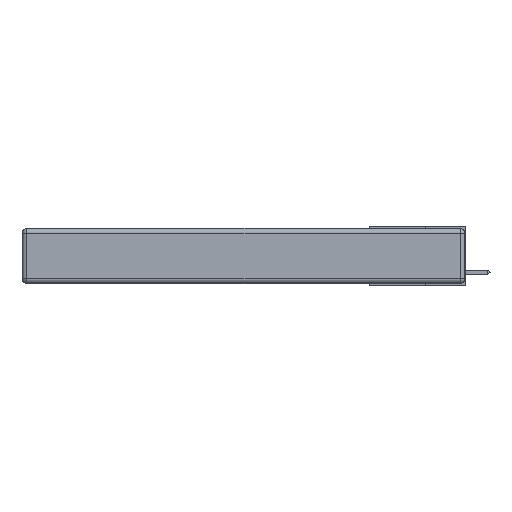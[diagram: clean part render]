
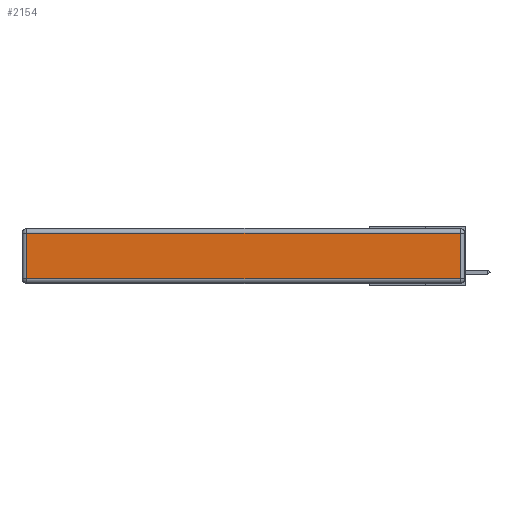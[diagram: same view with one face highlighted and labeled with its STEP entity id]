
A CAD part, left-side view. The second image highlights one B-rep face of the part: STEP entity #2154.
In plain terms, the highlighted planar face has unit normal (-1, 0, 0).
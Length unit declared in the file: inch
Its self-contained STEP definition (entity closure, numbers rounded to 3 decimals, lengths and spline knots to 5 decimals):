
#38 = CARTESIAN_POINT ( 'NONE',  ( 0., 2.75, -0.03 ) ) ;
#45 = CARTESIAN_POINT ( 'NONE',  ( 0., 0.03, -0.03 ) ) ;
#104 = DIRECTION ( 'NONE',  ( 0., 0., 1. ) ) ;
#1548 = VERTEX_POINT ( 'NONE', #6568 ) ;
#2064 = EDGE_LOOP ( 'NONE', ( #19879, #19993, #3849, #15967 ) ) ;
#2154 = ADVANCED_FACE ( 'NONE', ( #9152 ), #9570, .T. ) ;
#2314 = EDGE_CURVE ( 'NONE', #6201, #13058, #3477, .T. ) ;
#3466 = AXIS2_PLACEMENT_3D ( 'NONE', #19327, #9842, #104 ) ;
#3477 = LINE ( 'NONE', #8336, #7214 ) ;
#3849 = ORIENTED_EDGE ( 'NONE', *, *, #15371, .T. ) ;
#4821 = DIRECTION ( 'NONE',  ( 0., 1., 0. ) ) ;
#5034 = VECTOR ( 'NONE', #11539, 39.37008 ) ;
#6201 = VERTEX_POINT ( 'NONE', #10933 ) ;
#6568 = CARTESIAN_POINT ( 'NONE',  ( 0., 0.03, -0.313 ) ) ;
#7214 = VECTOR ( 'NONE', #10030, 39.37008 ) ;
#7406 = VECTOR ( 'NONE', #4821, 39.37008 ) ;
#8336 = CARTESIAN_POINT ( 'NONE',  ( 0., 2.72, -0.343 ) ) ;
#9152 = FACE_OUTER_BOUND ( 'NONE', #2064, .T. ) ;
#9570 = PLANE ( 'NONE',  #3466 ) ;
#9678 = VERTEX_POINT ( 'NONE', #45 ) ;
#9711 = LINE ( 'NONE', #13067, #5034 ) ;
#9842 = DIRECTION ( 'NONE',  ( -1., 0., 0. ) ) ;
#10030 = DIRECTION ( 'NONE',  ( 0., 0., -1. ) ) ;
#10848 = LINE ( 'NONE', #13841, #17559 ) ;
#10933 = CARTESIAN_POINT ( 'NONE',  ( 0., 2.72, -0.03 ) ) ;
#11539 = DIRECTION ( 'NONE',  ( 0., 0., 1. ) ) ;
#13058 = VERTEX_POINT ( 'NONE', #17441 ) ;
#13060 = LINE ( 'NONE', #38, #7406 ) ;
#13067 = CARTESIAN_POINT ( 'NONE',  ( 0., 0.03, -0.343 ) ) ;
#13841 = CARTESIAN_POINT ( 'NONE',  ( 0., 0., -0.313 ) ) ;
#14829 = EDGE_CURVE ( 'NONE', #13058, #1548, #10848, .T. ) ;
#15371 = EDGE_CURVE ( 'NONE', #9678, #6201, #13060, .T. ) ;
#15563 = DIRECTION ( 'NONE',  ( 0., -1., 0. ) ) ;
#15967 = ORIENTED_EDGE ( 'NONE', *, *, #2314, .T. ) ;
#17441 = CARTESIAN_POINT ( 'NONE',  ( 0., 2.72, -0.313 ) ) ;
#17559 = VECTOR ( 'NONE', #15563, 39.37008 ) ;
#18932 = EDGE_CURVE ( 'NONE', #1548, #9678, #9711, .T. ) ;
#19327 = CARTESIAN_POINT ( 'NONE',  ( 0., 0., -0.343 ) ) ;
#19879 = ORIENTED_EDGE ( 'NONE', *, *, #14829, .T. ) ;
#19993 = ORIENTED_EDGE ( 'NONE', *, *, #18932, .T. ) ;
